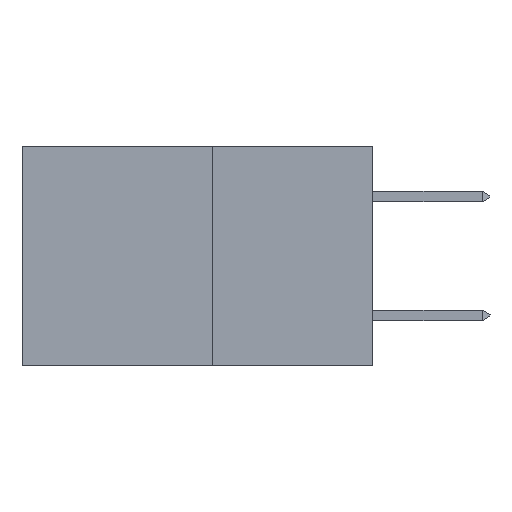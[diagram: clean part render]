
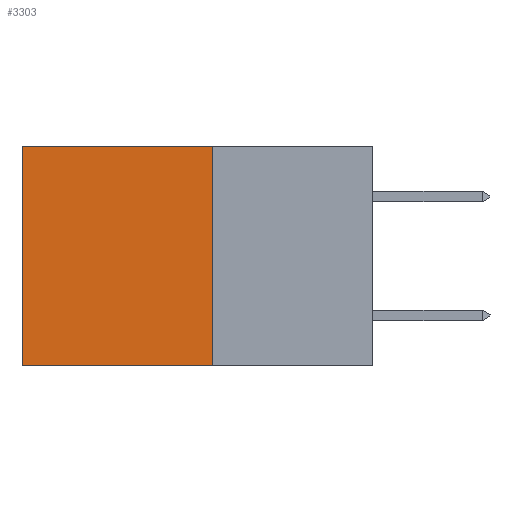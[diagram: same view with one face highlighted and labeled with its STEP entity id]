
A CAD part, left-side view. The second image highlights one B-rep face of the part: STEP entity #3303.
In plain terms, the highlighted planar face has unit normal (-1, 0, 0).
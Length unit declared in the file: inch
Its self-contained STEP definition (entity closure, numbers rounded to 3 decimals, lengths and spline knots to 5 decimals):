
#303 = CARTESIAN_POINT ( 'NONE',  ( 0.277, 0.27, 0. ) ) ;
#3303 = ADVANCED_FACE ( 'NONE', ( #8748 ), #34106, .F. ) ;
#4529 = VECTOR ( 'NONE', #16571, 39.37008 ) ;
#4645 = CARTESIAN_POINT ( 'NONE',  ( 0.277, 0.27, -0.37 ) ) ;
#4767 = DIRECTION ( 'NONE',  ( 0., 0., -1. ) ) ;
#4770 = CARTESIAN_POINT ( 'NONE',  ( 0.277, 0.27, -0.37 ) ) ;
#6069 = AXIS2_PLACEMENT_3D ( 'NONE', #23383, #14844, #6803 ) ;
#6803 = DIRECTION ( 'NONE',  ( 0., 0., -1. ) ) ;
#8583 = VECTOR ( 'NONE', #16057, 39.37008 ) ;
#8748 = FACE_OUTER_BOUND ( 'NONE', #14618, .T. ) ;
#10820 = VERTEX_POINT ( 'NONE', #16516 ) ;
#12489 = LINE ( 'NONE', #18119, #26716 ) ;
#13069 = VERTEX_POINT ( 'NONE', #17666 ) ;
#14618 = EDGE_LOOP ( 'NONE', ( #32113, #24057, #20653, #26963 ) ) ;
#14844 = DIRECTION ( 'NONE',  ( 1., 0., 0. ) ) ;
#14913 = LINE ( 'NONE', #31971, #8583 ) ;
#16057 = DIRECTION ( 'NONE',  ( 0., 1., 0. ) ) ;
#16516 = CARTESIAN_POINT ( 'NONE',  ( 0.277, 0.27, 0. ) ) ;
#16571 = DIRECTION ( 'NONE',  ( 0., 1., 0. ) ) ;
#17666 = CARTESIAN_POINT ( 'NONE',  ( 0.277, 0.59, 0. ) ) ;
#18119 = CARTESIAN_POINT ( 'NONE',  ( 0.277, 0.59, -0.37 ) ) ;
#18875 = LINE ( 'NONE', #303, #4529 ) ;
#20653 = ORIENTED_EDGE ( 'NONE', *, *, #21714, .F. ) ;
#20982 = VECTOR ( 'NONE', #4767, 39.37008 ) ;
#21714 = EDGE_CURVE ( 'NONE', #10820, #34042, #21830, .T. ) ;
#21830 = LINE ( 'NONE', #4645, #20982 ) ;
#21984 = EDGE_CURVE ( 'NONE', #10820, #13069, #18875, .T. ) ;
#22143 = VERTEX_POINT ( 'NONE', #30536 ) ;
#23383 = CARTESIAN_POINT ( 'NONE',  ( 0.277, 0.27, -0.37 ) ) ;
#24057 = ORIENTED_EDGE ( 'NONE', *, *, #25565, .F. ) ;
#25565 = EDGE_CURVE ( 'NONE', #34042, #22143, #14913, .T. ) ;
#26716 = VECTOR ( 'NONE', #34026, 39.37008 ) ;
#26963 = ORIENTED_EDGE ( 'NONE', *, *, #21984, .T. ) ;
#30536 = CARTESIAN_POINT ( 'NONE',  ( 0.277, 0.59, -0.37 ) ) ;
#31971 = CARTESIAN_POINT ( 'NONE',  ( 0.277, 0.27, -0.37 ) ) ;
#32113 = ORIENTED_EDGE ( 'NONE', *, *, #33381, .T. ) ;
#33381 = EDGE_CURVE ( 'NONE', #13069, #22143, #12489, .T. ) ;
#34026 = DIRECTION ( 'NONE',  ( 0., 0., -1. ) ) ;
#34042 = VERTEX_POINT ( 'NONE', #4770 ) ;
#34106 = PLANE ( 'NONE',  #6069 ) ;
